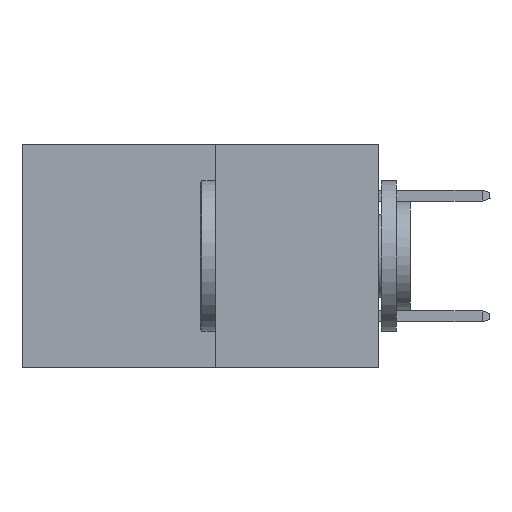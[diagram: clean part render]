
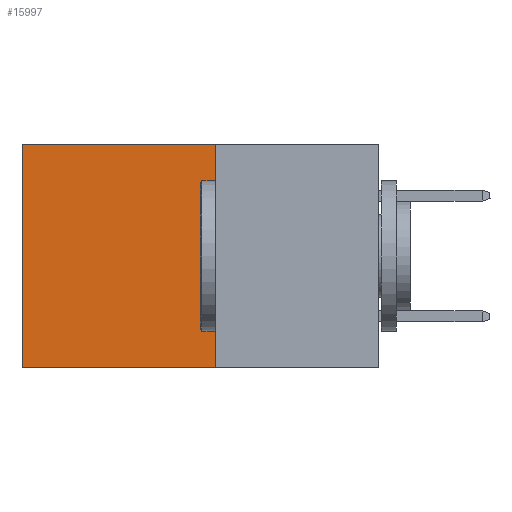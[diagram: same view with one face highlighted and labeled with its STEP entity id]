
A CAD part, left-side view. The second image highlights one B-rep face of the part: STEP entity #15997.
In plain terms, the highlighted planar face has unit normal (-1, 0, 0).
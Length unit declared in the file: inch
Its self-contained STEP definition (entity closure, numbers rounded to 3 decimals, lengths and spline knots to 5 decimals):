
#582 = ORIENTED_EDGE ( 'NONE', *, *, #6795, .F. ) ;
#1119 = CARTESIAN_POINT ( 'NONE',  ( 0.277, 0.59, -0.37 ) ) ;
#1447 = EDGE_CURVE ( 'NONE', #6679, #18413, #5959, .T. ) ;
#1732 = VECTOR ( 'NONE', #2199, 39.37008 ) ;
#1764 = EDGE_LOOP ( 'NONE', ( #3950, #9145, #582, #14163 ) ) ;
#2199 = DIRECTION ( 'NONE',  ( 0., 0., -1. ) ) ;
#2396 = CARTESIAN_POINT ( 'NONE',  ( 0.277, 0.27, 0. ) ) ;
#3827 = CARTESIAN_POINT ( 'NONE',  ( 0.277, 0.27, -0.37 ) ) ;
#3887 = DIRECTION ( 'NONE',  ( 0., 1., 0. ) ) ;
#3950 = ORIENTED_EDGE ( 'NONE', *, *, #1447, .T. ) ;
#4690 = PLANE ( 'NONE',  #19259 ) ;
#5135 = DIRECTION ( 'NONE',  ( 0., 1., 0. ) ) ;
#5562 = VERTEX_POINT ( 'NONE', #16481 ) ;
#5959 = LINE ( 'NONE', #1119, #1732 ) ;
#6211 = VECTOR ( 'NONE', #10166, 39.37008 ) ;
#6679 = VERTEX_POINT ( 'NONE', #6940 ) ;
#6795 = EDGE_CURVE ( 'NONE', #15688, #5562, #17338, .T. ) ;
#6940 = CARTESIAN_POINT ( 'NONE',  ( 0.277, 0.59, 0. ) ) ;
#7880 = DIRECTION ( 'NONE',  ( 0., 0., -1. ) ) ;
#9145 = ORIENTED_EDGE ( 'NONE', *, *, #16821, .F. ) ;
#9299 = LINE ( 'NONE', #17774, #13040 ) ;
#10166 = DIRECTION ( 'NONE',  ( 0., 0., -1. ) ) ;
#11062 = CARTESIAN_POINT ( 'NONE',  ( 0.277, 0.27, -0.37 ) ) ;
#13040 = VECTOR ( 'NONE', #5135, 39.37008 ) ;
#14163 = ORIENTED_EDGE ( 'NONE', *, *, #15470, .T. ) ;
#15470 = EDGE_CURVE ( 'NONE', #15688, #6679, #9299, .T. ) ;
#15688 = VERTEX_POINT ( 'NONE', #2396 ) ;
#15691 = FACE_OUTER_BOUND ( 'NONE', #1764, .T. ) ;
#15771 = CARTESIAN_POINT ( 'NONE',  ( 0.277, 0.27, -0.37 ) ) ;
#15997 = ADVANCED_FACE ( 'NONE', ( #15691 ), #4690, .F. ) ;
#16481 = CARTESIAN_POINT ( 'NONE',  ( 0.277, 0.27, -0.37 ) ) ;
#16622 = LINE ( 'NONE', #3827, #20363 ) ;
#16821 = EDGE_CURVE ( 'NONE', #5562, #18413, #16622, .T. ) ;
#17058 = CARTESIAN_POINT ( 'NONE',  ( 0.277, 0.59, -0.37 ) ) ;
#17338 = LINE ( 'NONE', #11062, #6211 ) ;
#17355 = DIRECTION ( 'NONE',  ( 1., 0., 0. ) ) ;
#17774 = CARTESIAN_POINT ( 'NONE',  ( 0.277, 0.27, 0. ) ) ;
#18413 = VERTEX_POINT ( 'NONE', #17058 ) ;
#19259 = AXIS2_PLACEMENT_3D ( 'NONE', #15771, #17355, #7880 ) ;
#20363 = VECTOR ( 'NONE', #3887, 39.37008 ) ;
